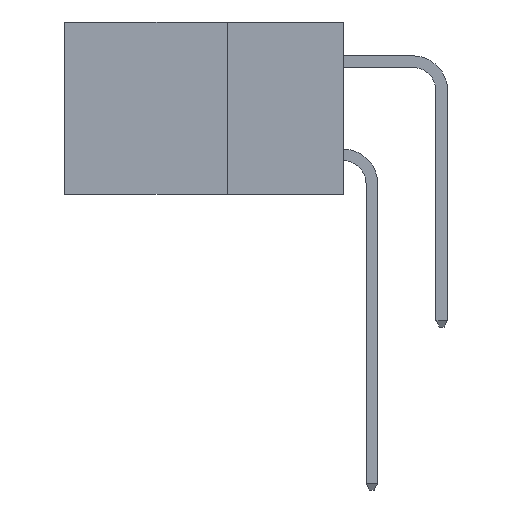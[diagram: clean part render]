
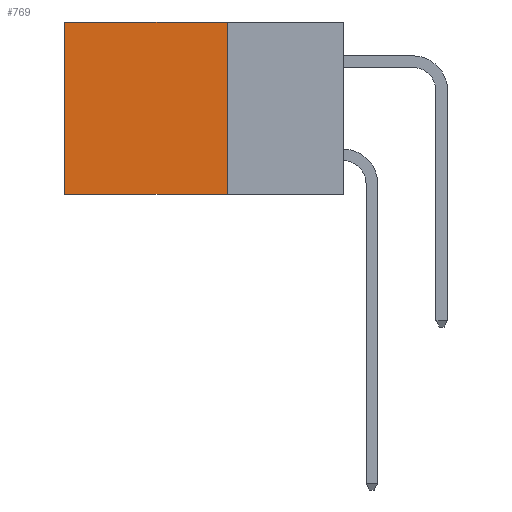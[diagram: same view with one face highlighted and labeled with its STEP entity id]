
A CAD part, left-side view. The second image highlights one B-rep face of the part: STEP entity #769.
In plain terms, the highlighted planar face has unit normal (-1, 0, 0).
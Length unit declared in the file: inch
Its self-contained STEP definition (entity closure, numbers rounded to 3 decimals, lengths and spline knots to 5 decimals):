
#769 = ADVANCED_FACE ( 'NONE', ( #15924 ), #12899, .F. ) ;
#1508 = CARTESIAN_POINT ( 'NONE',  ( 0.2615, 0.25, -0.37 ) ) ;
#1865 = LINE ( 'NONE', #16036, #9107 ) ;
#2162 = VERTEX_POINT ( 'NONE', #9385 ) ;
#2271 = CARTESIAN_POINT ( 'NONE',  ( 0.2615, 0.6, 0. ) ) ;
#2347 = EDGE_LOOP ( 'NONE', ( #15504, #8996, #14441, #14423 ) ) ;
#4185 = EDGE_CURVE ( 'NONE', #4522, #18459, #18501, .T. ) ;
#4522 = VERTEX_POINT ( 'NONE', #11200 ) ;
#5243 = VERTEX_POINT ( 'NONE', #2271 ) ;
#5250 = DIRECTION ( 'NONE',  ( 1., 0., 0. ) ) ;
#5514 = CARTESIAN_POINT ( 'NONE',  ( 0.2615, 0.25, -0.37 ) ) ;
#6174 = EDGE_CURVE ( 'NONE', #5243, #2162, #1865, .T. ) ;
#7185 = VECTOR ( 'NONE', #15842, 39.37008 ) ;
#7895 = LINE ( 'NONE', #11530, #11276 ) ;
#8720 = EDGE_CURVE ( 'NONE', #4522, #5243, #7895, .T. ) ;
#8996 = ORIENTED_EDGE ( 'NONE', *, *, #17569, .F. ) ;
#9107 = VECTOR ( 'NONE', #15932, 39.37008 ) ;
#9385 = CARTESIAN_POINT ( 'NONE',  ( 0.2615, 0.6, -0.37 ) ) ;
#10187 = DIRECTION ( 'NONE',  ( 0., 1., 0. ) ) ;
#11200 = CARTESIAN_POINT ( 'NONE',  ( 0.2615, 0.25, 0. ) ) ;
#11276 = VECTOR ( 'NONE', #11412, 39.37008 ) ;
#11412 = DIRECTION ( 'NONE',  ( 0., 1., 0. ) ) ;
#11473 = LINE ( 'NONE', #1508, #13465 ) ;
#11530 = CARTESIAN_POINT ( 'NONE',  ( 0.2615, 0.25, 0. ) ) ;
#12448 = AXIS2_PLACEMENT_3D ( 'NONE', #5514, #5250, #15917 ) ;
#12899 = PLANE ( 'NONE',  #12448 ) ;
#13465 = VECTOR ( 'NONE', #10187, 39.37008 ) ;
#13638 = CARTESIAN_POINT ( 'NONE',  ( 0.2615, 0.25, -0.37 ) ) ;
#14423 = ORIENTED_EDGE ( 'NONE', *, *, #8720, .T. ) ;
#14441 = ORIENTED_EDGE ( 'NONE', *, *, #4185, .F. ) ;
#15504 = ORIENTED_EDGE ( 'NONE', *, *, #6174, .T. ) ;
#15675 = CARTESIAN_POINT ( 'NONE',  ( 0.2615, 0.25, -0.37 ) ) ;
#15842 = DIRECTION ( 'NONE',  ( 0., 0., -1. ) ) ;
#15917 = DIRECTION ( 'NONE',  ( 0., 0., -1. ) ) ;
#15924 = FACE_OUTER_BOUND ( 'NONE', #2347, .T. ) ;
#15932 = DIRECTION ( 'NONE',  ( 0., 0., -1. ) ) ;
#16036 = CARTESIAN_POINT ( 'NONE',  ( 0.2615, 0.6, -0.37 ) ) ;
#17569 = EDGE_CURVE ( 'NONE', #18459, #2162, #11473, .T. ) ;
#18459 = VERTEX_POINT ( 'NONE', #13638 ) ;
#18501 = LINE ( 'NONE', #15675, #7185 ) ;
